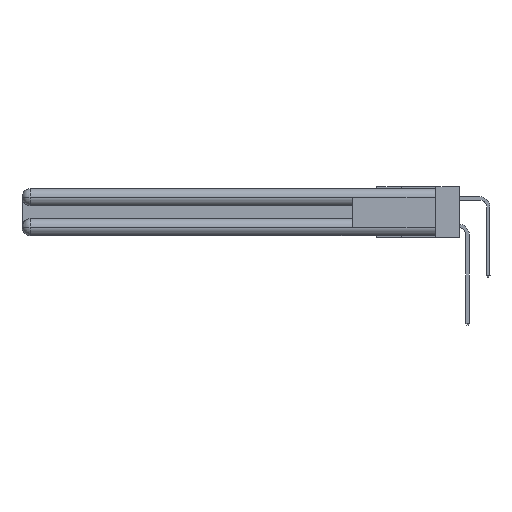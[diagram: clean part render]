
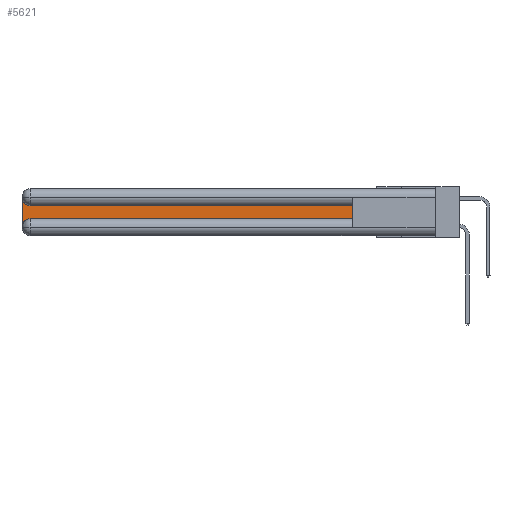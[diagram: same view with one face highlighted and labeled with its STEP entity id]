
A CAD part, left-side view. The second image highlights one B-rep face of the part: STEP entity #5621.
In plain terms, the highlighted planar face has unit normal (-1, 0, 0).
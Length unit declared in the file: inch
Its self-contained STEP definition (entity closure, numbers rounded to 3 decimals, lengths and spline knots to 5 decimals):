
#1186 = PLANE ( 'NONE',  #17315 ) ;
#1328 = CARTESIAN_POINT ( 'NONE',  ( 0.075, 3., -0.2775 ) ) ;
#1465 = ORIENTED_EDGE ( 'NONE', *, *, #24931, .T. ) ;
#1492 = VECTOR ( 'NONE', #7088, 39.37008 ) ;
#3230 = ORIENTED_EDGE ( 'NONE', *, *, #23184, .T. ) ;
#3330 = DIRECTION ( 'NONE',  ( 0., -1., 0. ) ) ;
#3692 = CARTESIAN_POINT ( 'NONE',  ( 0.075, 3., -0.1225 ) ) ;
#3809 = DIRECTION ( 'NONE',  ( 1., 0., 0. ) ) ;
#4015 = CARTESIAN_POINT ( 'NONE',  ( 0.075, 2.94, -0.0625 ) ) ;
#4034 = VERTEX_POINT ( 'NONE', #24833 ) ;
#4252 = AXIS2_PLACEMENT_3D ( 'NONE', #6799, #23905, #23806 ) ;
#4793 = EDGE_LOOP ( 'NONE', ( #3230, #10584, #12160, #16442, #15846, #1465 ) ) ;
#5273 = DIRECTION ( 'NONE',  ( 1., 0., 0. ) ) ;
#5621 = ADVANCED_FACE ( 'NONE', ( #17081 ), #1186, .F. ) ;
#6183 = DIRECTION ( 'NONE',  ( 0., 0., -1. ) ) ;
#6707 = VERTEX_POINT ( 'NONE', #30048 ) ;
#6799 = CARTESIAN_POINT ( 'NONE',  ( 0.075, 2.94, -0.2775 ) ) ;
#7088 = DIRECTION ( 'NONE',  ( 0., 0., 1. ) ) ;
#7200 = AXIS2_PLACEMENT_3D ( 'NONE', #4015, #5273, #16090 ) ;
#7308 = LINE ( 'NONE', #19228, #1492 ) ;
#9130 = VERTEX_POINT ( 'NONE', #1328 ) ;
#9209 = EDGE_CURVE ( 'NONE', #4034, #30101, #12096, .T. ) ;
#10415 = VERTEX_POINT ( 'NONE', #18391 ) ;
#10584 = ORIENTED_EDGE ( 'NONE', *, *, #9209, .T. ) ;
#10795 = CARTESIAN_POINT ( 'NONE',  ( 0.075, 3., -0.0625 ) ) ;
#11957 = LINE ( 'NONE', #20227, #30852 ) ;
#12096 = CIRCLE ( 'NONE', #7200, 0.06 ) ;
#12160 = ORIENTED_EDGE ( 'NONE', *, *, #31557, .T. ) ;
#14432 = DIRECTION ( 'NONE',  ( 0., 0., -1. ) ) ;
#15812 = VECTOR ( 'NONE', #14432, 39.37008 ) ;
#15846 = ORIENTED_EDGE ( 'NONE', *, *, #18514, .T. ) ;
#16090 = DIRECTION ( 'NONE',  ( 0., 0., -1. ) ) ;
#16442 = ORIENTED_EDGE ( 'NONE', *, *, #30354, .T. ) ;
#16852 = DIRECTION ( 'NONE',  ( 0., 1., 0. ) ) ;
#17081 = FACE_OUTER_BOUND ( 'NONE', #4793, .T. ) ;
#17315 = AXIS2_PLACEMENT_3D ( 'NONE', #3692, #3809, #6183 ) ;
#17355 = LINE ( 'NONE', #26379, #15812 ) ;
#17498 = CARTESIAN_POINT ( 'NONE',  ( 0.075, 0.6, -0.1225 ) ) ;
#18391 = CARTESIAN_POINT ( 'NONE',  ( 0.075, 2.94, -0.2175 ) ) ;
#18514 = EDGE_CURVE ( 'NONE', #10415, #6707, #11957, .T. ) ;
#19228 = CARTESIAN_POINT ( 'NONE',  ( 0.075, 0.6, -0.2175 ) ) ;
#19775 = CIRCLE ( 'NONE', #4252, 0.06 ) ;
#20227 = CARTESIAN_POINT ( 'NONE',  ( 0.075, 0.6, -0.2175 ) ) ;
#23184 = EDGE_CURVE ( 'NONE', #26600, #4034, #28593, .T. ) ;
#23806 = DIRECTION ( 'NONE',  ( 0., 0., -1. ) ) ;
#23905 = DIRECTION ( 'NONE',  ( 1., 0., 0. ) ) ;
#24833 = CARTESIAN_POINT ( 'NONE',  ( 0.075, 2.94, -0.1225 ) ) ;
#24931 = EDGE_CURVE ( 'NONE', #6707, #26600, #7308, .T. ) ;
#26379 = CARTESIAN_POINT ( 'NONE',  ( 0.075, 3., -0.2175 ) ) ;
#26600 = VERTEX_POINT ( 'NONE', #17498 ) ;
#28593 = LINE ( 'NONE', #31756, #30538 ) ;
#30048 = CARTESIAN_POINT ( 'NONE',  ( 0.075, 0.6, -0.2175 ) ) ;
#30101 = VERTEX_POINT ( 'NONE', #10795 ) ;
#30354 = EDGE_CURVE ( 'NONE', #9130, #10415, #19775, .T. ) ;
#30538 = VECTOR ( 'NONE', #16852, 39.37008 ) ;
#30852 = VECTOR ( 'NONE', #3330, 39.37008 ) ;
#31557 = EDGE_CURVE ( 'NONE', #30101, #9130, #17355, .T. ) ;
#31756 = CARTESIAN_POINT ( 'NONE',  ( 0.075, 0.6, -0.1225 ) ) ;
